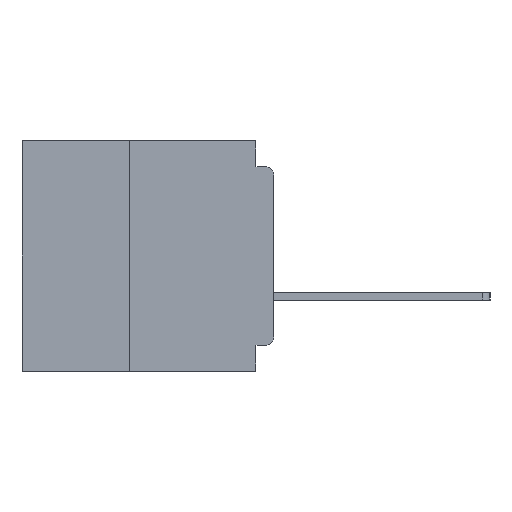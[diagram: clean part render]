
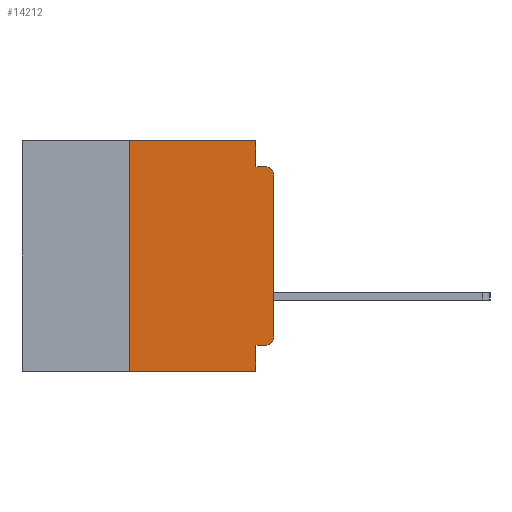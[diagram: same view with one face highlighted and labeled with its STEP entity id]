
A CAD part, left-side view. The second image highlights one B-rep face of the part: STEP entity #14212.
In plain terms, the highlighted planar face has unit normal (-1, 0, 0).
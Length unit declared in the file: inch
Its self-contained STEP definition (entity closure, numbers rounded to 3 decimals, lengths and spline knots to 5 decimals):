
#15 = CARTESIAN_POINT ( 'NONE',  ( 0., 0.437, 0. ) ) ;
#125 = DIRECTION ( 'NONE',  ( -1., 0., 0. ) ) ;
#141 = ORIENTED_EDGE ( 'NONE', *, *, #19558, .T. ) ;
#437 = VERTEX_POINT ( 'NONE', #16022 ) ;
#511 = DIRECTION ( 'NONE',  ( 0., 0., -1. ) ) ;
#1001 = ORIENTED_EDGE ( 'NONE', *, *, #4161, .T. ) ;
#1246 = ORIENTED_EDGE ( 'NONE', *, *, #21432, .F. ) ;
#1358 = CARTESIAN_POINT ( 'NONE',  ( 0., 0., -0.355 ) ) ;
#1594 = CARTESIAN_POINT ( 'NONE',  ( 0., 0.031, -0.045 ) ) ;
#1854 = LINE ( 'NONE', #20066, #44114 ) ;
#1889 = CARTESIAN_POINT ( 'NONE',  ( 0., 0., 0. ) ) ;
#2574 = CARTESIAN_POINT ( 'NONE',  ( 0., 0.25, -0.4 ) ) ;
#2830 = ORIENTED_EDGE ( 'NONE', *, *, #47175, .F. ) ;
#2999 = ORIENTED_EDGE ( 'NONE', *, *, #50068, .F. ) ;
#3576 = ORIENTED_EDGE ( 'NONE', *, *, #29289, .F. ) ;
#4161 = EDGE_CURVE ( 'NONE', #8236, #437, #45195, .T. ) ;
#4323 = ORIENTED_EDGE ( 'NONE', *, *, #22592, .T. ) ;
#4624 = ORIENTED_EDGE ( 'NONE', *, *, #14784, .F. ) ;
#4661 = VECTOR ( 'NONE', #34710, 39.37008 ) ;
#5609 = ORIENTED_EDGE ( 'NONE', *, *, #19498, .F. ) ;
#5761 = ORIENTED_EDGE ( 'NONE', *, *, #6818, .T. ) ;
#5788 = VERTEX_POINT ( 'NONE', #20762 ) ;
#6818 = EDGE_CURVE ( 'NONE', #7746, #5788, #21977, .T. ) ;
#7746 = VERTEX_POINT ( 'NONE', #38942 ) ;
#8236 = VERTEX_POINT ( 'NONE', #45036 ) ;
#9966 = LINE ( 'NONE', #50821, #42603 ) ;
#10670 = AXIS2_PLACEMENT_3D ( 'NONE', #24832, #125, #28897 ) ;
#12426 = CARTESIAN_POINT ( 'NONE',  ( 0., 0.031, -0.4 ) ) ;
#14212 = ADVANCED_FACE ( 'NONE', ( #40163 ), #45114, .F. ) ;
#14784 = EDGE_CURVE ( 'NONE', #14906, #36270, #20625, .T. ) ;
#14906 = VERTEX_POINT ( 'NONE', #50245 ) ;
#15213 = CARTESIAN_POINT ( 'NONE',  ( 0., 0.015, -0.06 ) ) ;
#16022 = CARTESIAN_POINT ( 'NONE',  ( 0., 0.015, -0.045 ) ) ;
#17878 = VECTOR ( 'NONE', #23107, 39.37008 ) ;
#19371 = DIRECTION ( 'NONE',  ( 0., 0., -1. ) ) ;
#19498 = EDGE_CURVE ( 'NONE', #7746, #14906, #20792, .T. ) ;
#19558 = EDGE_CURVE ( 'NONE', #5788, #8236, #26596, .T. ) ;
#20066 = CARTESIAN_POINT ( 'NONE',  ( 0., 0.031, 0. ) ) ;
#20437 = VECTOR ( 'NONE', #26205, 39.37008 ) ;
#20625 = LINE ( 'NONE', #25215, #41025 ) ;
#20730 = DIRECTION ( 'NONE',  ( 1., 0., 0. ) ) ;
#20762 = CARTESIAN_POINT ( 'NONE',  ( 0., 0., -0.34 ) ) ;
#20792 = LINE ( 'NONE', #1358, #39932 ) ;
#21432 = EDGE_CURVE ( 'NONE', #34703, #437, #52929, .T. ) ;
#21977 = CIRCLE ( 'NONE', #10670, 0.015 ) ;
#22592 = EDGE_CURVE ( 'NONE', #25689, #36270, #37545, .T. ) ;
#23107 = DIRECTION ( 'NONE',  ( 0., 0., 1. ) ) ;
#24832 = CARTESIAN_POINT ( 'NONE',  ( 0., 0.015, -0.34 ) ) ;
#25215 = CARTESIAN_POINT ( 'NONE',  ( 0., 0.031, -0.4 ) ) ;
#25443 = EDGE_LOOP ( 'NONE', ( #141, #1001, #1246, #2830, #2999, #3576, #4323, #4624, #5609, #5761 ) ) ;
#25689 = VERTEX_POINT ( 'NONE', #41084 ) ;
#26205 = DIRECTION ( 'NONE',  ( 0., -1., 0. ) ) ;
#26504 = DIRECTION ( 'NONE',  ( 0., -1., 0. ) ) ;
#26596 = LINE ( 'NONE', #1889, #4661 ) ;
#28897 = DIRECTION ( 'NONE',  ( 0., 0., -1. ) ) ;
#29289 = EDGE_CURVE ( 'NONE', #25689, #29318, #50378, .T. ) ;
#29318 = VERTEX_POINT ( 'NONE', #51737 ) ;
#30094 = DIRECTION ( 'NONE',  ( 0., 1., 0. ) ) ;
#31880 = AXIS2_PLACEMENT_3D ( 'NONE', #15213, #43756, #19371 ) ;
#34703 = VERTEX_POINT ( 'NONE', #1594 ) ;
#34710 = DIRECTION ( 'NONE',  ( 0., 0., 1. ) ) ;
#36262 = VECTOR ( 'NONE', #46962, 39.37008 ) ;
#36270 = VERTEX_POINT ( 'NONE', #12426 ) ;
#37545 = LINE ( 'NONE', #42887, #36262 ) ;
#38271 = CARTESIAN_POINT ( 'NONE',  ( 0., 0., -0.045 ) ) ;
#38942 = CARTESIAN_POINT ( 'NONE',  ( 0., 0.015, -0.355 ) ) ;
#39932 = VECTOR ( 'NONE', #30094, 39.37008 ) ;
#40163 = FACE_OUTER_BOUND ( 'NONE', #25443, .T. ) ;
#41025 = VECTOR ( 'NONE', #511, 39.37008 ) ;
#41084 = CARTESIAN_POINT ( 'NONE',  ( 0., 0.25, -0.4 ) ) ;
#42603 = VECTOR ( 'NONE', #26504, 39.37008 ) ;
#42887 = CARTESIAN_POINT ( 'NONE',  ( 0., 0.437, -0.4 ) ) ;
#43756 = DIRECTION ( 'NONE',  ( -1., 0., 0. ) ) ;
#44114 = VECTOR ( 'NONE', #48575, 39.37008 ) ;
#45036 = CARTESIAN_POINT ( 'NONE',  ( 0., 0., -0.06 ) ) ;
#45114 = PLANE ( 'NONE',  #48227 ) ;
#45195 = CIRCLE ( 'NONE', #31880, 0.015 ) ;
#46962 = DIRECTION ( 'NONE',  ( 0., -1., 0. ) ) ;
#47175 = EDGE_CURVE ( 'NONE', #51680, #34703, #1854, .T. ) ;
#48227 = AXIS2_PLACEMENT_3D ( 'NONE', #15, #20730, #49224 ) ;
#48575 = DIRECTION ( 'NONE',  ( 0., 0., -1. ) ) ;
#49224 = DIRECTION ( 'NONE',  ( 0., 0., -1. ) ) ;
#50068 = EDGE_CURVE ( 'NONE', #29318, #51680, #9966, .T. ) ;
#50245 = CARTESIAN_POINT ( 'NONE',  ( 0., 0.031, -0.355 ) ) ;
#50378 = LINE ( 'NONE', #2574, #17878 ) ;
#50821 = CARTESIAN_POINT ( 'NONE',  ( 0., 0.437, 0. ) ) ;
#51680 = VERTEX_POINT ( 'NONE', #52552 ) ;
#51737 = CARTESIAN_POINT ( 'NONE',  ( 0., 0.25, 0. ) ) ;
#52552 = CARTESIAN_POINT ( 'NONE',  ( 0., 0.031, 0. ) ) ;
#52929 = LINE ( 'NONE', #38271, #20437 ) ;
